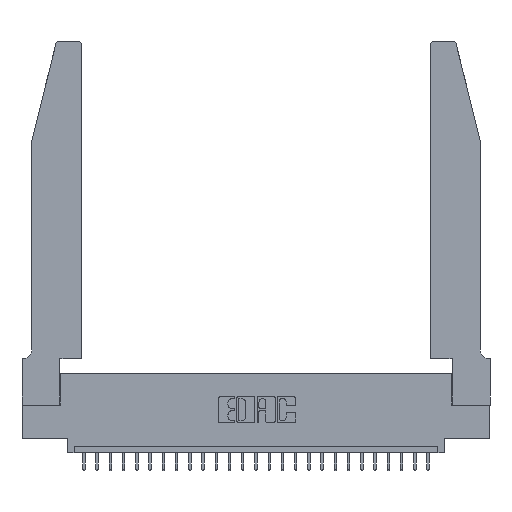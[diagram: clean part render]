
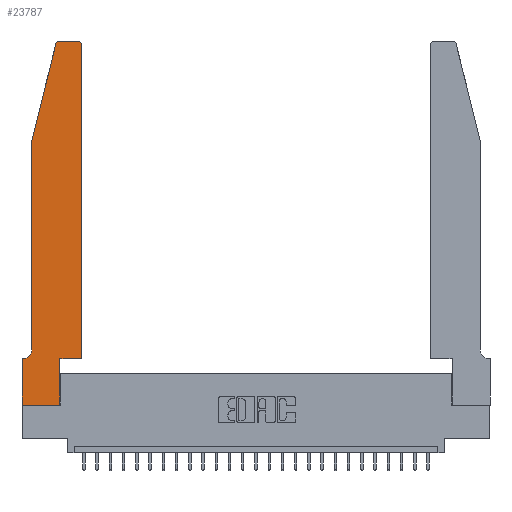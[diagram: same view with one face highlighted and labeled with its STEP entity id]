
A CAD part, top view. The second image highlights one B-rep face of the part: STEP entity #23787.
In plain terms, the highlighted planar face has unit normal (0, 0, 1).
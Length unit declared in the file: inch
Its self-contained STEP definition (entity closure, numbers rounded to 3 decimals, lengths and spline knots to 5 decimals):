
#178 = DIRECTION ( 'NONE',  ( 1., 0., 0. ) ) ;
#210 = ORIENTED_EDGE ( 'NONE', *, *, #13930, .T. ) ;
#1099 = VERTEX_POINT ( 'NONE', #21190 ) ;
#1415 = VECTOR ( 'NONE', #20515, 39.37008 ) ;
#1614 = EDGE_CURVE ( 'NONE', #2182, #26800, #9150, .T. ) ;
#1662 = CARTESIAN_POINT ( 'NONE',  ( 0.2865, 0., 0.37 ) ) ;
#1771 = VERTEX_POINT ( 'NONE', #19821 ) ;
#2182 = VERTEX_POINT ( 'NONE', #8748 ) ;
#2618 = VERTEX_POINT ( 'NONE', #2738 ) ;
#2738 = CARTESIAN_POINT ( 'NONE',  ( 0.4505, 2.72, 0.37 ) ) ;
#2941 = VECTOR ( 'NONE', #12458, 39.37008 ) ;
#4150 = CARTESIAN_POINT ( 'NONE',  ( 0.4505, 0.35, 0.37 ) ) ;
#4239 = ORIENTED_EDGE ( 'NONE', *, *, #11043, .T. ) ;
#4286 = ORIENTED_EDGE ( 'NONE', *, *, #26185, .T. ) ;
#4588 = ORIENTED_EDGE ( 'NONE', *, *, #7098, .T. ) ;
#4808 = CARTESIAN_POINT ( 'NONE',  ( 0.0755, 0.35, 0.37 ) ) ;
#4940 = LINE ( 'NONE', #4808, #11868 ) ;
#6957 = ORIENTED_EDGE ( 'NONE', *, *, #26200, .T. ) ;
#7062 = ORIENTED_EDGE ( 'NONE', *, *, #15819, .T. ) ;
#7098 = EDGE_CURVE ( 'NONE', #15237, #2618, #19096, .T. ) ;
#7133 = CARTESIAN_POINT ( 'NONE',  ( 0.284, 2.72, 0.37 ) ) ;
#7274 = VERTEX_POINT ( 'NONE', #1662 ) ;
#8279 = CARTESIAN_POINT ( 'NONE',  ( 0.4505, 0.35, 0.37 ) ) ;
#8288 = AXIS2_PLACEMENT_3D ( 'NONE', #18448, #14037, #16393 ) ;
#8748 = CARTESIAN_POINT ( 'NONE',  ( 0.0755, 0.42, 0.37 ) ) ;
#8833 = DIRECTION ( 'NONE',  ( -1., 0., 0. ) ) ;
#9150 = CIRCLE ( 'NONE', #8288, 0.07 ) ;
#9593 = CARTESIAN_POINT ( 'NONE',  ( 0.4205, 2.75, 0.37 ) ) ;
#9707 = VERTEX_POINT ( 'NONE', #16696 ) ;
#10070 = CARTESIAN_POINT ( 'NONE',  ( 0., 0., 0.37 ) ) ;
#10199 = VERTEX_POINT ( 'NONE', #25372 ) ;
#10321 = CARTESIAN_POINT ( 'NONE',  ( 0.25487, 2.72718, 0.37 ) ) ;
#10655 = CARTESIAN_POINT ( 'NONE',  ( 0., 0.35, 0.37 ) ) ;
#10945 = ORIENTED_EDGE ( 'NONE', *, *, #16341, .T. ) ;
#10972 = AXIS2_PLACEMENT_3D ( 'NONE', #7133, #17231, #23481 ) ;
#11043 = EDGE_CURVE ( 'NONE', #1771, #7274, #23357, .T. ) ;
#11068 = PLANE ( 'NONE',  #26362 ) ;
#11089 = EDGE_CURVE ( 'NONE', #26800, #9707, #4940, .T. ) ;
#11138 = LINE ( 'NONE', #13351, #21132 ) ;
#11451 = VECTOR ( 'NONE', #19187, 39.37008 ) ;
#11470 = ORIENTED_EDGE ( 'NONE', *, *, #18153, .T. ) ;
#11668 = VERTEX_POINT ( 'NONE', #17040 ) ;
#11868 = VECTOR ( 'NONE', #8833, 39.37008 ) ;
#12458 = DIRECTION ( 'NONE',  ( 0., 1., 0. ) ) ;
#12494 = DIRECTION ( 'NONE',  ( -1., 0., 0. ) ) ;
#12550 = LINE ( 'NONE', #20996, #11451 ) ;
#12562 = LINE ( 'NONE', #18935, #25270 ) ;
#13184 = EDGE_LOOP ( 'NONE', ( #22127, #4286, #210, #6957, #15087, #15029, #15877, #4239, #7062, #10945, #4588, #11470 ) ) ;
#13351 = CARTESIAN_POINT ( 'NONE',  ( 0.0755, 2., 0.37 ) ) ;
#13930 = EDGE_CURVE ( 'NONE', #15553, #11668, #12550, .T. ) ;
#14037 = DIRECTION ( 'NONE',  ( 0., 0., -1. ) ) ;
#14086 = VERTEX_POINT ( 'NONE', #9593 ) ;
#14526 = CIRCLE ( 'NONE', #10972, 0.03 ) ;
#14687 = CARTESIAN_POINT ( 'NONE',  ( 0.0055, 0.35, 0.37 ) ) ;
#14771 = DIRECTION ( 'NONE',  ( 1., 0., 0. ) ) ;
#15029 = ORIENTED_EDGE ( 'NONE', *, *, #11089, .T. ) ;
#15087 = ORIENTED_EDGE ( 'NONE', *, *, #1614, .T. ) ;
#15237 = VERTEX_POINT ( 'NONE', #8279 ) ;
#15364 = DIRECTION ( 'NONE',  ( 0., 0., 1. ) ) ;
#15405 = VECTOR ( 'NONE', #14771, 39.37008 ) ;
#15553 = VERTEX_POINT ( 'NONE', #10321 ) ;
#15819 = EDGE_CURVE ( 'NONE', #7274, #1099, #26341, .T. ) ;
#15877 = ORIENTED_EDGE ( 'NONE', *, *, #19352, .T. ) ;
#15942 = EDGE_CURVE ( 'NONE', #14086, #10199, #16505, .T. ) ;
#15965 = CARTESIAN_POINT ( 'NONE',  ( 0.2865, 0.35, 0.37 ) ) ;
#16341 = EDGE_CURVE ( 'NONE', #1099, #15237, #12562, .T. ) ;
#16393 = DIRECTION ( 'NONE',  ( -1., 0., 0. ) ) ;
#16505 = LINE ( 'NONE', #17159, #26137 ) ;
#16696 = CARTESIAN_POINT ( 'NONE',  ( 0., 0.35, 0.37 ) ) ;
#17040 = CARTESIAN_POINT ( 'NONE',  ( 0.0755, 2., 0.37 ) ) ;
#17070 = DIRECTION ( 'NONE',  ( 1., 0., 0. ) ) ;
#17159 = CARTESIAN_POINT ( 'NONE',  ( 0.2605, 2.75, 0.37 ) ) ;
#17231 = DIRECTION ( 'NONE',  ( 0., 0., 1. ) ) ;
#18153 = EDGE_CURVE ( 'NONE', #2618, #14086, #27086, .T. ) ;
#18448 = CARTESIAN_POINT ( 'NONE',  ( 0.0055, 0.42, 0.37 ) ) ;
#18892 = DIRECTION ( 'NONE',  ( 0., -1., 0. ) ) ;
#18935 = CARTESIAN_POINT ( 'NONE',  ( 0.4505, 0.35, 0.37 ) ) ;
#19096 = LINE ( 'NONE', #4150, #2941 ) ;
#19187 = DIRECTION ( 'NONE',  ( -0.239, -0.971, 0. ) ) ;
#19352 = EDGE_CURVE ( 'NONE', #9707, #1771, #25121, .T. ) ;
#19703 = DIRECTION ( 'NONE',  ( 0., -1., 0. ) ) ;
#19821 = CARTESIAN_POINT ( 'NONE',  ( 0., 0., 0.37 ) ) ;
#20515 = DIRECTION ( 'NONE',  ( 0., 1., 0. ) ) ;
#20996 = CARTESIAN_POINT ( 'NONE',  ( 0.0755, 2., 0.37 ) ) ;
#21132 = VECTOR ( 'NONE', #19703, 39.37008 ) ;
#21190 = CARTESIAN_POINT ( 'NONE',  ( 0.2865, 0.35, 0.37 ) ) ;
#22127 = ORIENTED_EDGE ( 'NONE', *, *, #15942, .T. ) ;
#23177 = CARTESIAN_POINT ( 'NONE',  ( 0.4205, 2.72, 0.37 ) ) ;
#23183 = CARTESIAN_POINT ( 'NONE',  ( 0., 0., 0.37 ) ) ;
#23357 = LINE ( 'NONE', #10070, #15405 ) ;
#23460 = DIRECTION ( 'NONE',  ( 0., 0., 1. ) ) ;
#23481 = DIRECTION ( 'NONE',  ( 1., 0., 0. ) ) ;
#23590 = VECTOR ( 'NONE', #18892, 39.37008 ) ;
#23787 = ADVANCED_FACE ( 'NONE', ( #25870 ), #11068, .T. ) ;
#25121 = LINE ( 'NONE', #23183, #23590 ) ;
#25270 = VECTOR ( 'NONE', #25427, 39.37008 ) ;
#25372 = CARTESIAN_POINT ( 'NONE',  ( 0.284, 2.75, 0.37 ) ) ;
#25427 = DIRECTION ( 'NONE',  ( 1., 0., 0. ) ) ;
#25870 = FACE_OUTER_BOUND ( 'NONE', #13184, .T. ) ;
#26137 = VECTOR ( 'NONE', #12494, 39.37008 ) ;
#26185 = EDGE_CURVE ( 'NONE', #10199, #15553, #14526, .T. ) ;
#26200 = EDGE_CURVE ( 'NONE', #11668, #2182, #11138, .T. ) ;
#26214 = AXIS2_PLACEMENT_3D ( 'NONE', #23177, #23460, #17070 ) ;
#26341 = LINE ( 'NONE', #15965, #1415 ) ;
#26362 = AXIS2_PLACEMENT_3D ( 'NONE', #10655, #15364, #178 ) ;
#26800 = VERTEX_POINT ( 'NONE', #14687 ) ;
#27086 = CIRCLE ( 'NONE', #26214, 0.03 ) ;
